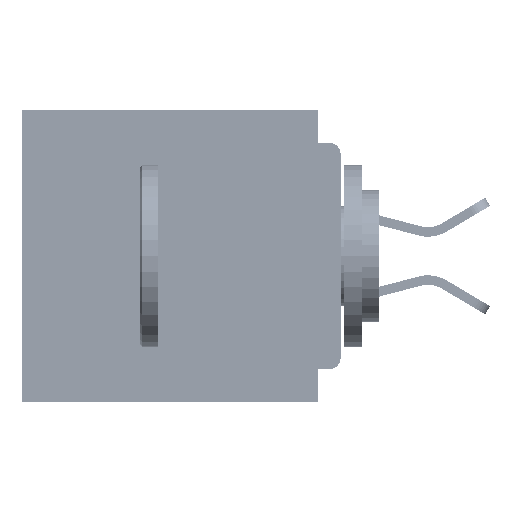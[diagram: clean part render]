
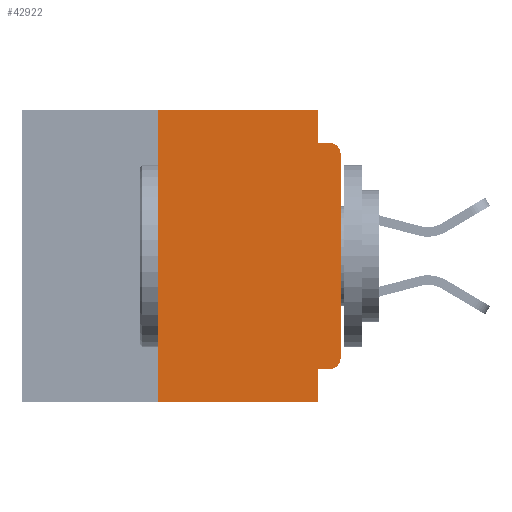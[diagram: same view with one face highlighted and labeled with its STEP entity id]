
A CAD part, left-side view. The second image highlights one B-rep face of the part: STEP entity #42922.
In plain terms, the highlighted planar face has unit normal (-1, 0, 0).
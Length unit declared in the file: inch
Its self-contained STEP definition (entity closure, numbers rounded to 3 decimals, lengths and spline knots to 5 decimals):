
#518 = CARTESIAN_POINT ( 'NONE',  ( 0., 0., -0.34 ) ) ;
#1537 = VERTEX_POINT ( 'NONE', #25853 ) ;
#2331 = VECTOR ( 'NONE', #52082, 39.37008 ) ;
#3387 = LINE ( 'NONE', #52353, #23597 ) ;
#3975 = DIRECTION ( 'NONE',  ( 0., 0., -1. ) ) ;
#5739 = CARTESIAN_POINT ( 'NONE',  ( 0., 0.25, -0.4 ) ) ;
#7550 = CARTESIAN_POINT ( 'NONE',  ( 0., 0.437, -0.4 ) ) ;
#8101 = CARTESIAN_POINT ( 'NONE',  ( 0., 0.031, -0.045 ) ) ;
#8226 = CIRCLE ( 'NONE', #33097, 0.015 ) ;
#8471 = ORIENTED_EDGE ( 'NONE', *, *, #43329, .F. ) ;
#8970 = DIRECTION ( 'NONE',  ( 0., 0., -1. ) ) ;
#9885 = CARTESIAN_POINT ( 'NONE',  ( 0., 0., -0.355 ) ) ;
#10466 = VERTEX_POINT ( 'NONE', #47941 ) ;
#10949 = LINE ( 'NONE', #35750, #51438 ) ;
#11219 = VECTOR ( 'NONE', #39700, 39.37008 ) ;
#11378 = VERTEX_POINT ( 'NONE', #50667 ) ;
#12291 = DIRECTION ( 'NONE',  ( 0., -1., 0. ) ) ;
#12473 = ORIENTED_EDGE ( 'NONE', *, *, #38377, .T. ) ;
#14567 = EDGE_CURVE ( 'NONE', #45008, #52127, #30842, .T. ) ;
#14587 = DIRECTION ( 'NONE',  ( 0., 0., 1. ) ) ;
#15992 = CARTESIAN_POINT ( 'NONE',  ( 0., 0.015, -0.06 ) ) ;
#16502 = DIRECTION ( 'NONE',  ( 0., 0., 1. ) ) ;
#16686 = CARTESIAN_POINT ( 'NONE',  ( 0., 0.015, -0.34 ) ) ;
#17540 = VECTOR ( 'NONE', #14587, 39.37008 ) ;
#18187 = EDGE_LOOP ( 'NONE', ( #46140, #50035, #39577, #19409, #8471, #37529, #30986, #19776, #51537, #12473 ) ) ;
#19371 = CARTESIAN_POINT ( 'NONE',  ( 0., 0.437, 0. ) ) ;
#19409 = ORIENTED_EDGE ( 'NONE', *, *, #25779, .F. ) ;
#19776 = ORIENTED_EDGE ( 'NONE', *, *, #50149, .F. ) ;
#20041 = DIRECTION ( 'NONE',  ( 0., 0., -1. ) ) ;
#20088 = CARTESIAN_POINT ( 'NONE',  ( 0., 0., -0.06 ) ) ;
#20723 = DIRECTION ( 'NONE',  ( 0., 0., -1. ) ) ;
#21202 = EDGE_CURVE ( 'NONE', #37803, #1537, #8226, .T. ) ;
#21254 = EDGE_CURVE ( 'NONE', #47145, #1537, #46170, .T. ) ;
#21960 = LINE ( 'NONE', #19371, #11219 ) ;
#22617 = VECTOR ( 'NONE', #38148, 39.37008 ) ;
#23273 = EDGE_CURVE ( 'NONE', #33084, #10466, #25052, .T. ) ;
#23597 = VECTOR ( 'NONE', #3975, 39.37008 ) ;
#23617 = CARTESIAN_POINT ( 'NONE',  ( 0., 0.031, -0.355 ) ) ;
#23672 = AXIS2_PLACEMENT_3D ( 'NONE', #16686, #44986, #20723 ) ;
#23814 = AXIS2_PLACEMENT_3D ( 'NONE', #49239, #33160, #8970 ) ;
#25052 = LINE ( 'NONE', #7550, #2331 ) ;
#25779 = EDGE_CURVE ( 'NONE', #41465, #47145, #3387, .T. ) ;
#25853 = CARTESIAN_POINT ( 'NONE',  ( 0., 0.015, -0.045 ) ) ;
#28965 = FACE_OUTER_BOUND ( 'NONE', #18187, .T. ) ;
#29647 = VECTOR ( 'NONE', #16502, 39.37008 ) ;
#30842 = LINE ( 'NONE', #9885, #22617 ) ;
#30986 = ORIENTED_EDGE ( 'NONE', *, *, #23273, .T. ) ;
#33084 = VERTEX_POINT ( 'NONE', #5739 ) ;
#33097 = AXIS2_PLACEMENT_3D ( 'NONE', #15992, #44284, #20041 ) ;
#33160 = DIRECTION ( 'NONE',  ( 1., 0., 0. ) ) ;
#33838 = CIRCLE ( 'NONE', #23672, 0.015 ) ;
#34477 = EDGE_CURVE ( 'NONE', #42331, #37803, #39068, .T. ) ;
#35386 = VECTOR ( 'NONE', #12291, 39.37008 ) ;
#35412 = CARTESIAN_POINT ( 'NONE',  ( 0., 0.031, 0. ) ) ;
#35750 = CARTESIAN_POINT ( 'NONE',  ( 0., 0.031, -0.4 ) ) ;
#36654 = CARTESIAN_POINT ( 'NONE',  ( 0., 0.25, -0.4 ) ) ;
#37529 = ORIENTED_EDGE ( 'NONE', *, *, #51622, .F. ) ;
#37803 = VERTEX_POINT ( 'NONE', #20088 ) ;
#37851 = LINE ( 'NONE', #36654, #29647 ) ;
#38148 = DIRECTION ( 'NONE',  ( 0., 1., 0. ) ) ;
#38377 = EDGE_CURVE ( 'NONE', #45008, #42331, #33838, .T. ) ;
#38799 = CARTESIAN_POINT ( 'NONE',  ( 0., 0., 0. ) ) ;
#39068 = LINE ( 'NONE', #38799, #17540 ) ;
#39577 = ORIENTED_EDGE ( 'NONE', *, *, #21254, .F. ) ;
#39700 = DIRECTION ( 'NONE',  ( 0., -1., 0. ) ) ;
#41118 = PLANE ( 'NONE',  #23814 ) ;
#41465 = VERTEX_POINT ( 'NONE', #35412 ) ;
#42331 = VERTEX_POINT ( 'NONE', #518 ) ;
#42922 = ADVANCED_FACE ( 'NONE', ( #28965 ), #41118, .F. ) ;
#43329 = EDGE_CURVE ( 'NONE', #11378, #41465, #21960, .T. ) ;
#44284 = DIRECTION ( 'NONE',  ( -1., 0., 0. ) ) ;
#44458 = CARTESIAN_POINT ( 'NONE',  ( 0., 0., -0.045 ) ) ;
#44986 = DIRECTION ( 'NONE',  ( -1., 0., 0. ) ) ;
#45008 = VERTEX_POINT ( 'NONE', #50897 ) ;
#46140 = ORIENTED_EDGE ( 'NONE', *, *, #34477, .T. ) ;
#46170 = LINE ( 'NONE', #44458, #35386 ) ;
#47145 = VERTEX_POINT ( 'NONE', #8101 ) ;
#47941 = CARTESIAN_POINT ( 'NONE',  ( 0., 0.031, -0.4 ) ) ;
#49239 = CARTESIAN_POINT ( 'NONE',  ( 0., 0.437, 0. ) ) ;
#50035 = ORIENTED_EDGE ( 'NONE', *, *, #21202, .T. ) ;
#50149 = EDGE_CURVE ( 'NONE', #52127, #10466, #10949, .T. ) ;
#50667 = CARTESIAN_POINT ( 'NONE',  ( 0., 0.25, 0. ) ) ;
#50897 = CARTESIAN_POINT ( 'NONE',  ( 0., 0.015, -0.355 ) ) ;
#51438 = VECTOR ( 'NONE', #51832, 39.37008 ) ;
#51537 = ORIENTED_EDGE ( 'NONE', *, *, #14567, .F. ) ;
#51622 = EDGE_CURVE ( 'NONE', #33084, #11378, #37851, .T. ) ;
#51832 = DIRECTION ( 'NONE',  ( 0., 0., -1. ) ) ;
#52082 = DIRECTION ( 'NONE',  ( 0., -1., 0. ) ) ;
#52127 = VERTEX_POINT ( 'NONE', #23617 ) ;
#52353 = CARTESIAN_POINT ( 'NONE',  ( 0., 0.031, 0. ) ) ;
